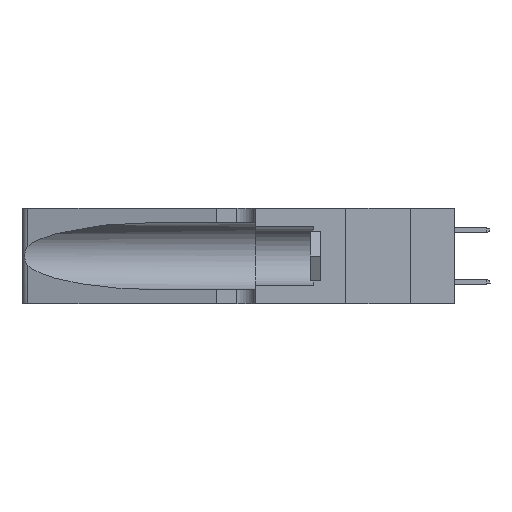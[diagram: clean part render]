
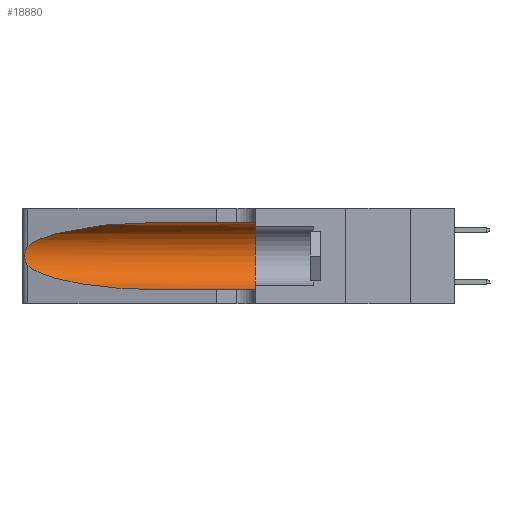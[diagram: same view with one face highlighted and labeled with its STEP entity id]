
A CAD part, left-side view. The second image highlights one B-rep face of the part: STEP entity #18880.
In plain terms, the highlighted cylindrical face has radius 3.308 mm (diameter 6.617 mm), a partial arc.
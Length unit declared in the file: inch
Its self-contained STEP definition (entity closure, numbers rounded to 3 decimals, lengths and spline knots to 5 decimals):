
#549 = CARTESIAN_POINT ( 'NONE',  ( 0.25487, 1.22718, 0.14631 ) ) ;
#728 = CARTESIAN_POINT ( 'NONE',  ( 0.25555, 1.22994, 0.2215 ) ) ;
#769 = CARTESIAN_POINT ( 'NONE',  ( 0.25555, 1.22993, 0.14849 ) ) ;
#889 = CARTESIAN_POINT ( 'NONE',  ( 0.25854, 1.2359, 0.20912 ) ) ;
#947 = LINE ( 'NONE', #18595, #13041 ) ;
#1179 = CARTESIAN_POINT ( 'NONE',  ( 0.1305, 0.72297, 0.05475 ) ) ;
#1839 = EDGE_CURVE ( 'NONE', #8727, #22295, #6879, .T. ) ;
#2183 = ORIENTED_EDGE ( 'NONE', *, *, #18350, .F. ) ;
#2730 = CARTESIAN_POINT ( 'NONE',  ( 0.25789, 1.23486, 0.15765 ) ) ;
#3072 = CARTESIAN_POINT ( 'NONE',  ( 0.25487, 1.22718, 0.22369 ) ) ;
#4297 = VECTOR ( 'NONE', #17789, 39.37008 ) ;
#4678 = DIRECTION ( 'NONE',  ( 0., 1., 0. ) ) ;
#4911 = CARTESIAN_POINT ( 'NONE',  ( 0.25856, 1.23593, 0.16098 ) ) ;
#5216 = EDGE_CURVE ( 'NONE', #12835, #8727, #25483, .T. ) ;
#6351 = ORIENTED_EDGE ( 'NONE', *, *, #1839, .T. ) ;
#6560 = CARTESIAN_POINT ( 'NONE',  ( 0.25487, 1.22718, 0.22369 ) ) ;
#6728 = ORIENTED_EDGE ( 'NONE', *, *, #5216, .T. ) ;
#6729 = CARTESIAN_POINT ( 'NONE',  ( 0.26075, 1.23896, 0.178 ) ) ;
#6861 = CARTESIAN_POINT ( 'NONE',  ( 0.26017, 1.23833, 0.17102 ) ) ;
#6879 =( BOUNDED_CURVE ( )  B_SPLINE_CURVE ( 3, ( #549, #16102, #10560, #15985 ),
 .UNSPECIFIED., .F., .T. ) 
 B_SPLINE_CURVE_WITH_KNOTS ( ( 4, 4 ),
 ( 3.44316, 4.71239 ),
 .UNSPECIFIED. ) 
 CURVE ( )  GEOMETRIC_REPRESENTATION_ITEM ( )  RATIONAL_B_SPLINE_CURVE ( ( 1., 0.87, 0.87, 1. ) ) 
 REPRESENTATION_ITEM ( '' )  );
#6889 = CARTESIAN_POINT ( 'NONE',  ( 0.25487, 1.22718, 0.22369 ) ) ;
#7300 = EDGE_CURVE ( 'NONE', #15620, #22838, #21684, .T. ) ;
#8202 = EDGE_CURVE ( 'NONE', #22295, #24896, #947, .T. ) ;
#8727 = VERTEX_POINT ( 'NONE', #16226 ) ;
#9606 = ORIENTED_EDGE ( 'NONE', *, *, #17370, .T. ) ;
#10366 = CARTESIAN_POINT ( 'NONE',  ( 0.1305, 0.35, 0.31525 ) ) ;
#10560 = CARTESIAN_POINT ( 'NONE',  ( 0.18966, 0.96281, 0.05475 ) ) ;
#10628 = CARTESIAN_POINT ( 'NONE',  ( 0.1305, 1.61858, 0.185 ) ) ;
#10655 = CARTESIAN_POINT ( 'NONE',  ( 0.25639, 1.23186, 0.15144 ) ) ;
#11451 = AXIS2_PLACEMENT_3D ( 'NONE', #10628, #24582, #14875 ) ;
#12656 = DIRECTION ( 'NONE',  ( 0., -1., 0. ) ) ;
#12835 = VERTEX_POINT ( 'NONE', #6889 ) ;
#13041 = VECTOR ( 'NONE', #12656, 39.37008 ) ;
#13331 = CARTESIAN_POINT ( 'NONE',  ( 0.18966, 0.96281, 0.31525 ) ) ;
#13479 = AXIS2_PLACEMENT_3D ( 'NONE', #20126, #4678, #14536 ) ;
#14536 = DIRECTION ( 'NONE',  ( 0., 0., 1. ) ) ;
#14875 = DIRECTION ( 'NONE',  ( 0., 0., -1. ) ) ;
#14993 =( BOUNDED_CURVE ( )  B_SPLINE_CURVE ( 3, ( #20842, #13331, #15264, #3072 ),
 .UNSPECIFIED., .F., .T. ) 
 B_SPLINE_CURVE_WITH_KNOTS ( ( 4, 4 ),
 ( 1.5708, 2.84003 ),
 .UNSPECIFIED. ) 
 CURVE ( )  GEOMETRIC_REPRESENTATION_ITEM ( )  RATIONAL_B_SPLINE_CURVE ( ( 1., 0.87, 0.87, 1. ) ) 
 REPRESENTATION_ITEM ( '' )  );
#15264 = CARTESIAN_POINT ( 'NONE',  ( 0.2373, 1.15595, 0.28018 ) ) ;
#15620 = VERTEX_POINT ( 'NONE', #22555 ) ;
#15985 = CARTESIAN_POINT ( 'NONE',  ( 0.1305, 0.72297, 0.05475 ) ) ;
#16102 = CARTESIAN_POINT ( 'NONE',  ( 0.2373, 1.15595, 0.08982 ) ) ;
#16226 = CARTESIAN_POINT ( 'NONE',  ( 0.25487, 1.22718, 0.14631 ) ) ;
#16692 = ORIENTED_EDGE ( 'NONE', *, *, #7300, .F. ) ;
#16710 = CARTESIAN_POINT ( 'NONE',  ( 0.26075, 1.23896, 0.19203 ) ) ;
#17370 = EDGE_CURVE ( 'NONE', #15620, #12835, #14993, .T. ) ;
#17789 = DIRECTION ( 'NONE',  ( 0., -1., 0. ) ) ;
#18350 = EDGE_CURVE ( 'NONE', #22838, #24896, #24615, .T. ) ;
#18547 = CARTESIAN_POINT ( 'NONE',  ( 0.25487, 1.22718, 0.14631 ) ) ;
#18595 = CARTESIAN_POINT ( 'NONE',  ( 0.1305, 1.61858, 0.05475 ) ) ;
#18880 = ADVANCED_FACE ( 'NONE', ( #22648 ), #19027, .F. ) ;
#19027 = CYLINDRICAL_SURFACE ( 'NONE', #11451, 0.13025 ) ;
#19752 = CARTESIAN_POINT ( 'NONE',  ( 0.1305, 1.61858, 0.31525 ) ) ;
#20030 = EDGE_LOOP ( 'NONE', ( #9606, #6728, #6351, #22030, #2183, #16692 ) ) ;
#20126 = CARTESIAN_POINT ( 'NONE',  ( 0.1305, 0.35, 0.185 ) ) ;
#20461 = CARTESIAN_POINT ( 'NONE',  ( 0.25787, 1.23484, 0.2124 ) ) ;
#20842 = CARTESIAN_POINT ( 'NONE',  ( 0.1305, 0.72297, 0.31525 ) ) ;
#21684 = LINE ( 'NONE', #19752, #4297 ) ;
#22030 = ORIENTED_EDGE ( 'NONE', *, *, #8202, .T. ) ;
#22295 = VERTEX_POINT ( 'NONE', #1179 ) ;
#22555 = CARTESIAN_POINT ( 'NONE',  ( 0.1305, 0.72297, 0.31525 ) ) ;
#22648 = FACE_OUTER_BOUND ( 'NONE', #20030, .T. ) ;
#22674 = CARTESIAN_POINT ( 'NONE',  ( 0.26018, 1.23835, 0.19895 ) ) ;
#22838 = VERTEX_POINT ( 'NONE', #10366 ) ;
#23893 = CARTESIAN_POINT ( 'NONE',  ( 0.1305, 0.35, 0.05475 ) ) ;
#24315 = CARTESIAN_POINT ( 'NONE',  ( 0.25639, 1.23184, 0.21858 ) ) ;
#24582 = DIRECTION ( 'NONE',  ( 0., -1., 0. ) ) ;
#24615 = CIRCLE ( 'NONE', #13479, 0.13025 ) ;
#24896 = VERTEX_POINT ( 'NONE', #23893 ) ;
#25483 = B_SPLINE_CURVE_WITH_KNOTS ( 'NONE', 3,
 ( #6560, #728, #24315, #20461, #889, #22674, #16710, #6729, #6861, #4911, #2730, #10655, #769, #18547 ),
 .UNSPECIFIED., .F., .F.,
 ( 4, 2, 2, 2, 2, 2, 4 ),
 ( 0., 0.00027, 0.00053, 0.00107, 0.0016, 0.00187, 0.00214 ),
 .UNSPECIFIED. ) ;
